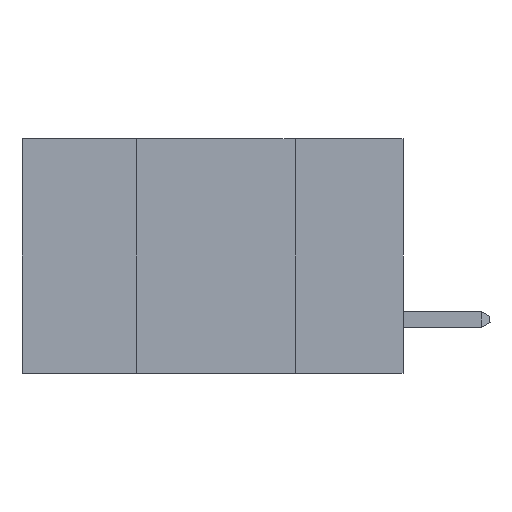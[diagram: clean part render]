
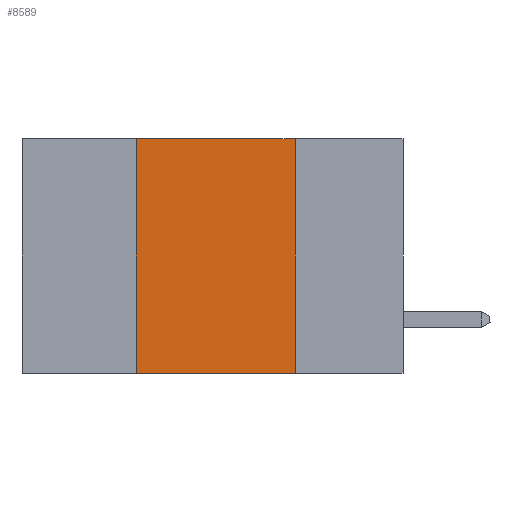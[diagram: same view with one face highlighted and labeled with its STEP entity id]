
A CAD part, left-side view. The second image highlights one B-rep face of the part: STEP entity #8589.
In plain terms, the highlighted planar face has unit normal (-1, 0, 0).
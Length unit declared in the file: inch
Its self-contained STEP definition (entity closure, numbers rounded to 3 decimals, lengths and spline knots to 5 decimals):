
#606 = DIRECTION ( 'NONE',  ( 0., -1., 0. ) ) ;
#645 = VECTOR ( 'NONE', #18472, 39.37008 ) ;
#970 = EDGE_CURVE ( 'NONE', #6924, #14565, #20594, .T. ) ;
#1465 = ORIENTED_EDGE ( 'NONE', *, *, #11643, .F. ) ;
#3095 = ORIENTED_EDGE ( 'NONE', *, *, #10956, .F. ) ;
#3540 = CARTESIAN_POINT ( 'NONE',  ( 0., 0.42, 0. ) ) ;
#3625 = DIRECTION ( 'NONE',  ( 0., 0., 1. ) ) ;
#5449 = CARTESIAN_POINT ( 'NONE',  ( 0., 0.6, 0. ) ) ;
#5514 = CARTESIAN_POINT ( 'NONE',  ( 0., 0.17, 0. ) ) ;
#6047 = FACE_OUTER_BOUND ( 'NONE', #18397, .T. ) ;
#6924 = VERTEX_POINT ( 'NONE', #5514 ) ;
#7481 = DIRECTION ( 'NONE',  ( 0., -1., 0. ) ) ;
#8589 = ADVANCED_FACE ( 'NONE', ( #6047 ), #9428, .F. ) ;
#9138 = VERTEX_POINT ( 'NONE', #14539 ) ;
#9428 = PLANE ( 'NONE',  #21459 ) ;
#9539 = VECTOR ( 'NONE', #7481, 39.37008 ) ;
#10956 = EDGE_CURVE ( 'NONE', #14920, #6924, #21760, .T. ) ;
#11384 = DIRECTION ( 'NONE',  ( 1., 0., 0. ) ) ;
#11643 = EDGE_CURVE ( 'NONE', #9138, #14920, #12331, .T. ) ;
#12331 = LINE ( 'NONE', #3540, #20254 ) ;
#14237 = ORIENTED_EDGE ( 'NONE', *, *, #970, .F. ) ;
#14539 = CARTESIAN_POINT ( 'NONE',  ( 0., 0.42, -0.37 ) ) ;
#14565 = VERTEX_POINT ( 'NONE', #21450 ) ;
#14920 = VERTEX_POINT ( 'NONE', #16045 ) ;
#15007 = ORIENTED_EDGE ( 'NONE', *, *, #15031, .T. ) ;
#15031 = EDGE_CURVE ( 'NONE', #9138, #14565, #23327, .T. ) ;
#16045 = CARTESIAN_POINT ( 'NONE',  ( 0., 0.42, 0. ) ) ;
#16592 = CARTESIAN_POINT ( 'NONE',  ( 0., 0.17, 0. ) ) ;
#18397 = EDGE_LOOP ( 'NONE', ( #14237, #3095, #1465, #15007 ) ) ;
#18472 = DIRECTION ( 'NONE',  ( 0., 0., -1. ) ) ;
#18547 = DIRECTION ( 'NONE',  ( 0., 0., -1. ) ) ;
#19366 = CARTESIAN_POINT ( 'NONE',  ( 0., 0.6, 0. ) ) ;
#20002 = VECTOR ( 'NONE', #606, 39.37008 ) ;
#20254 = VECTOR ( 'NONE', #3625, 39.37008 ) ;
#20594 = LINE ( 'NONE', #16592, #645 ) ;
#21069 = CARTESIAN_POINT ( 'NONE',  ( 0., 0.6, -0.37 ) ) ;
#21450 = CARTESIAN_POINT ( 'NONE',  ( 0., 0.17, -0.37 ) ) ;
#21459 = AXIS2_PLACEMENT_3D ( 'NONE', #5449, #11384, #18547 ) ;
#21760 = LINE ( 'NONE', #19366, #20002 ) ;
#23327 = LINE ( 'NONE', #21069, #9539 ) ;
